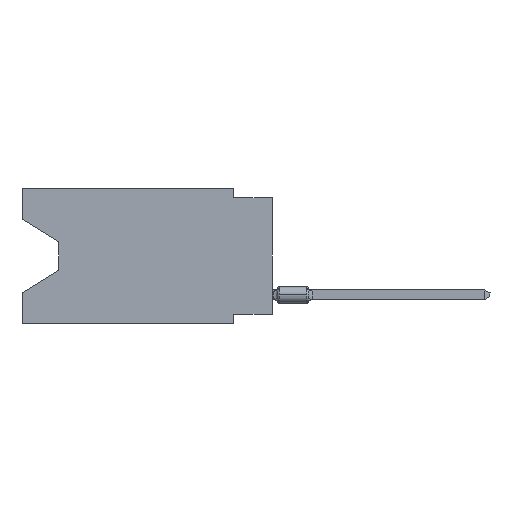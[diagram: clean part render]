
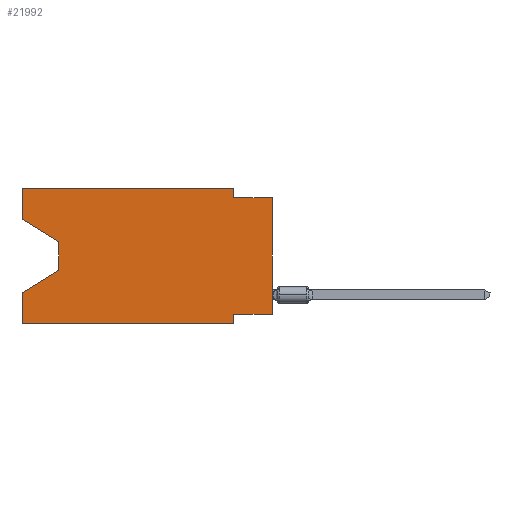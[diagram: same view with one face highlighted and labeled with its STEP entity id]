
A CAD part, left-side view. The second image highlights one B-rep face of the part: STEP entity #21992.
In plain terms, the highlighted planar face has unit normal (-1, 0, 0).
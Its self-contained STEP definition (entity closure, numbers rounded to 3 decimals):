
#1613 = ORIENTED_EDGE ( 'NONE', *, *, #7720, .T. ) ;
#4415 = LINE ( 'NONE', #65432, #39687 ) ;
#4449 = CARTESIAN_POINT ( 'NONE',  ( 0., 0., -8.255 ) ) ;
#7669 = EDGE_CURVE ( 'NONE', #103486, #106816, #89164, .T. ) ;
#7720 = EDGE_CURVE ( 'NONE', #61450, #28025, #72228, .T. ) ;
#10315 = LINE ( 'NONE', #87184, #45250 ) ;
#10675 = VERTEX_POINT ( 'NONE', #105591 ) ;
#12307 = CARTESIAN_POINT ( 'NONE',  ( 0., 16.383, -8.89 ) ) ;
#15441 = PLANE ( 'NONE',  #55538 ) ;
#15474 = VECTOR ( 'NONE', #89724, 1000. ) ;
#15544 = VECTOR ( 'NONE', #83575, 1000. ) ;
#15674 = EDGE_CURVE ( 'NONE', #26058, #93423, #97725, .T. ) ;
#16564 = DIRECTION ( 'NONE',  ( 0., 0., -1. ) ) ;
#16721 = VERTEX_POINT ( 'NONE', #49192 ) ;
#21992 = ADVANCED_FACE ( 'NONE', ( #109275 ), #15441, .F. ) ;
#23022 = LINE ( 'NONE', #57503, #111755 ) ;
#24777 = CARTESIAN_POINT ( 'NONE',  ( 0., 16.383, -2.038 ) ) ;
#24828 = EDGE_CURVE ( 'NONE', #10675, #103486, #10315, .T. ) ;
#26058 = VERTEX_POINT ( 'NONE', #75743 ) ;
#28025 = VERTEX_POINT ( 'NONE', #66210 ) ;
#28315 = CARTESIAN_POINT ( 'NONE',  ( 0., 13.97, -5.385 ) ) ;
#29041 = EDGE_CURVE ( 'NONE', #106816, #16721, #35235, .T. ) ;
#29324 = DIRECTION ( 'NONE',  ( 0., 0., -1. ) ) ;
#30698 = EDGE_LOOP ( 'NONE', ( #31145, #60491, #58536, #55349, #1613, #81921, #97851, #98999, #94602, #80234, #85946, #106270 ) ) ;
#31145 = ORIENTED_EDGE ( 'NONE', *, *, #55000, .T. ) ;
#34650 = LINE ( 'NONE', #60057, #87016 ) ;
#35235 = LINE ( 'NONE', #43173, #104364 ) ;
#36737 = CARTESIAN_POINT ( 'NONE',  ( 0., 2.54, -8.255 ) ) ;
#36802 = DIRECTION ( 'NONE',  ( 0., 0.855, -0.519 ) ) ;
#37152 = VECTOR ( 'NONE', #64810, 1000. ) ;
#39687 = VECTOR ( 'NONE', #57524, 1000. ) ;
#41462 = DIRECTION ( 'NONE',  ( 1., 0., 0. ) ) ;
#43173 = CARTESIAN_POINT ( 'NONE',  ( 0., 2.54, 0. ) ) ;
#43644 = LINE ( 'NONE', #88295, #51336 ) ;
#44268 = DIRECTION ( 'NONE',  ( 0., 0., -1. ) ) ;
#45250 = VECTOR ( 'NONE', #96222, 1000. ) ;
#45708 = EDGE_CURVE ( 'NONE', #93423, #108390, #61117, .T. ) ;
#46186 = LINE ( 'NONE', #63159, #37152 ) ;
#49192 = CARTESIAN_POINT ( 'NONE',  ( 0., 2.54, -0.635 ) ) ;
#51336 = VECTOR ( 'NONE', #86612, 1000. ) ;
#52115 = CARTESIAN_POINT ( 'NONE',  ( 0., 13.97, -5.385 ) ) ;
#55000 = EDGE_CURVE ( 'NONE', #10675, #26058, #102187, .T. ) ;
#55349 = ORIENTED_EDGE ( 'NONE', *, *, #77941, .F. ) ;
#55538 = AXIS2_PLACEMENT_3D ( 'NONE', #74252, #41462, #16564 ) ;
#57258 = CARTESIAN_POINT ( 'NONE',  ( 0., 16.383, -8.89 ) ) ;
#57503 = CARTESIAN_POINT ( 'NONE',  ( 0., 0., 0. ) ) ;
#57524 = DIRECTION ( 'NONE',  ( 0., 0., 1. ) ) ;
#58536 = ORIENTED_EDGE ( 'NONE', *, *, #45708, .T. ) ;
#60057 = CARTESIAN_POINT ( 'NONE',  ( 0., 0., -8.255 ) ) ;
#60491 = ORIENTED_EDGE ( 'NONE', *, *, #15674, .T. ) ;
#61117 = LINE ( 'NONE', #28315, #62356 ) ;
#61450 = VERTEX_POINT ( 'NONE', #57258 ) ;
#62356 = VECTOR ( 'NONE', #36802, 1000. ) ;
#62898 = EDGE_CURVE ( 'NONE', #79710, #82577, #34650, .T. ) ;
#63159 = CARTESIAN_POINT ( 'NONE',  ( 0., 0., -0.635 ) ) ;
#64810 = DIRECTION ( 'NONE',  ( 0., -1., 0. ) ) ;
#65432 = CARTESIAN_POINT ( 'NONE',  ( 0., 16.383, 0. ) ) ;
#66210 = CARTESIAN_POINT ( 'NONE',  ( 0., 2.54, -8.89 ) ) ;
#72228 = LINE ( 'NONE', #12307, #102115 ) ;
#74252 = CARTESIAN_POINT ( 'NONE',  ( 0., 16.383, 0. ) ) ;
#75743 = CARTESIAN_POINT ( 'NONE',  ( 0., 13.97, -3.505 ) ) ;
#76794 = EDGE_CURVE ( 'NONE', #79710, #107908, #23022, .T. ) ;
#77941 = EDGE_CURVE ( 'NONE', #61450, #108390, #4415, .T. ) ;
#78970 = CARTESIAN_POINT ( 'NONE',  ( 0., 16.383, -6.852 ) ) ;
#79710 = VERTEX_POINT ( 'NONE', #4449 ) ;
#79970 = CARTESIAN_POINT ( 'NONE',  ( 0., 0., -0.635 ) ) ;
#80234 = ORIENTED_EDGE ( 'NONE', *, *, #29041, .F. ) ;
#80561 = CARTESIAN_POINT ( 'NONE',  ( 0., 2.54, 0. ) ) ;
#80692 = DIRECTION ( 'NONE',  ( 0., -1., 0. ) ) ;
#81921 = ORIENTED_EDGE ( 'NONE', *, *, #108793, .F. ) ;
#82577 = VERTEX_POINT ( 'NONE', #36737 ) ;
#83575 = DIRECTION ( 'NONE',  ( 0., -0.855, -0.519 ) ) ;
#85946 = ORIENTED_EDGE ( 'NONE', *, *, #7669, .F. ) ;
#86612 = DIRECTION ( 'NONE',  ( 0., 0., -1. ) ) ;
#87016 = VECTOR ( 'NONE', #95108, 1000. ) ;
#87184 = CARTESIAN_POINT ( 'NONE',  ( 0., 16.383, 0. ) ) ;
#87504 = CARTESIAN_POINT ( 'NONE',  ( 0., 16.383, 0. ) ) ;
#88295 = CARTESIAN_POINT ( 'NONE',  ( 0., 2.54, -8.89 ) ) ;
#89164 = LINE ( 'NONE', #87504, #15474 ) ;
#89724 = DIRECTION ( 'NONE',  ( 0., -1., 0. ) ) ;
#91983 = DIRECTION ( 'NONE',  ( 0., 0., 1. ) ) ;
#92890 = VECTOR ( 'NONE', #29324, 1000. ) ;
#93423 = VERTEX_POINT ( 'NONE', #52115 ) ;
#94602 = ORIENTED_EDGE ( 'NONE', *, *, #99165, .F. ) ;
#95108 = DIRECTION ( 'NONE',  ( 0., 1., 0. ) ) ;
#96222 = DIRECTION ( 'NONE',  ( 0., 0., 1. ) ) ;
#97725 = LINE ( 'NONE', #104539, #92890 ) ;
#97851 = ORIENTED_EDGE ( 'NONE', *, *, #62898, .F. ) ;
#98623 = CARTESIAN_POINT ( 'NONE',  ( 0., 16.383, 0. ) ) ;
#98999 = ORIENTED_EDGE ( 'NONE', *, *, #76794, .T. ) ;
#99165 = EDGE_CURVE ( 'NONE', #16721, #107908, #46186, .T. ) ;
#102115 = VECTOR ( 'NONE', #80692, 1000. ) ;
#102187 = LINE ( 'NONE', #24777, #15544 ) ;
#103486 = VERTEX_POINT ( 'NONE', #98623 ) ;
#104364 = VECTOR ( 'NONE', #44268, 1000. ) ;
#104539 = CARTESIAN_POINT ( 'NONE',  ( 0., 13.97, -3.505 ) ) ;
#105591 = CARTESIAN_POINT ( 'NONE',  ( 0., 16.383, -2.038 ) ) ;
#106270 = ORIENTED_EDGE ( 'NONE', *, *, #24828, .F. ) ;
#106816 = VERTEX_POINT ( 'NONE', #80561 ) ;
#107908 = VERTEX_POINT ( 'NONE', #79970 ) ;
#108390 = VERTEX_POINT ( 'NONE', #78970 ) ;
#108793 = EDGE_CURVE ( 'NONE', #82577, #28025, #43644, .T. ) ;
#109275 = FACE_OUTER_BOUND ( 'NONE', #30698, .T. ) ;
#111755 = VECTOR ( 'NONE', #91983, 1000. ) ;
